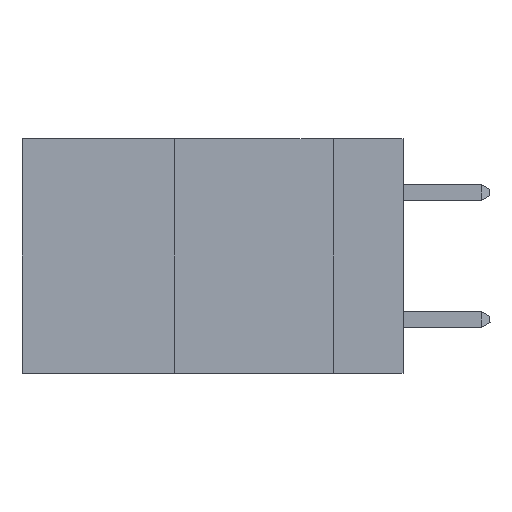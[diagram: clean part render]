
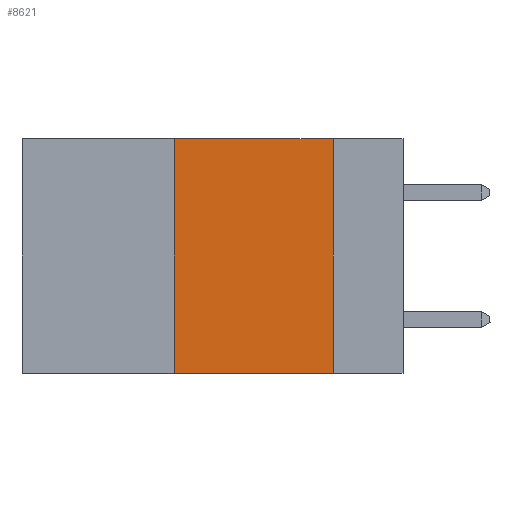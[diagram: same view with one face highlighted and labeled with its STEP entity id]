
A CAD part, left-side view. The second image highlights one B-rep face of the part: STEP entity #8621.
In plain terms, the highlighted planar face has unit normal (-1, 0, 0).
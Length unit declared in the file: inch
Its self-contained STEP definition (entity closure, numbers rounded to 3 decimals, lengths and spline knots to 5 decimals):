
#518 = PLANE ( 'NONE',  #20200 ) ;
#984 = DIRECTION ( 'NONE',  ( 0., 0., -1. ) ) ;
#2273 = VERTEX_POINT ( 'NONE', #17523 ) ;
#2694 = CARTESIAN_POINT ( 'NONE',  ( 0., 0.6, 0. ) ) ;
#3157 = ORIENTED_EDGE ( 'NONE', *, *, #17627, .T. ) ;
#3176 = EDGE_CURVE ( 'NONE', #18622, #2273, #8503, .T. ) ;
#4816 = DIRECTION ( 'NONE',  ( 0., 0., -1. ) ) ;
#5824 = EDGE_LOOP ( 'NONE', ( #12019, #20314, #16733, #3157 ) ) ;
#5862 = CARTESIAN_POINT ( 'NONE',  ( 0., 0.6, -0.37 ) ) ;
#7335 = LINE ( 'NONE', #13555, #12203 ) ;
#8503 = LINE ( 'NONE', #16429, #12730 ) ;
#8621 = ADVANCED_FACE ( 'NONE', ( #9488 ), #518, .F. ) ;
#9488 = FACE_OUTER_BOUND ( 'NONE', #5824, .T. ) ;
#10022 = VECTOR ( 'NONE', #26691, 39.37008 ) ;
#12019 = ORIENTED_EDGE ( 'NONE', *, *, #26061, .F. ) ;
#12203 = VECTOR ( 'NONE', #984, 39.37008 ) ;
#12730 = VECTOR ( 'NONE', #18592, 39.37008 ) ;
#13555 = CARTESIAN_POINT ( 'NONE',  ( 0., 0.11, 0. ) ) ;
#14818 = CARTESIAN_POINT ( 'NONE',  ( 0., 0.11, -0.37 ) ) ;
#15935 = VECTOR ( 'NONE', #19477, 39.37008 ) ;
#16429 = CARTESIAN_POINT ( 'NONE',  ( 0., 0.6, 0. ) ) ;
#16733 = ORIENTED_EDGE ( 'NONE', *, *, #23285, .F. ) ;
#17330 = DIRECTION ( 'NONE',  ( 1., 0., 0. ) ) ;
#17337 = CARTESIAN_POINT ( 'NONE',  ( 0., 0.36, 0. ) ) ;
#17523 = CARTESIAN_POINT ( 'NONE',  ( 0., 0.11, 0. ) ) ;
#17627 = EDGE_CURVE ( 'NONE', #23987, #26422, #26746, .T. ) ;
#18482 = CARTESIAN_POINT ( 'NONE',  ( 0., 0.36, 0. ) ) ;
#18592 = DIRECTION ( 'NONE',  ( 0., -1., 0. ) ) ;
#18622 = VERTEX_POINT ( 'NONE', #18482 ) ;
#19477 = DIRECTION ( 'NONE',  ( 0., 0., 1. ) ) ;
#19930 = CARTESIAN_POINT ( 'NONE',  ( 0., 0.36, -0.37 ) ) ;
#20200 = AXIS2_PLACEMENT_3D ( 'NONE', #2694, #17330, #4816 ) ;
#20314 = ORIENTED_EDGE ( 'NONE', *, *, #3176, .F. ) ;
#23285 = EDGE_CURVE ( 'NONE', #23987, #18622, #27087, .T. ) ;
#23987 = VERTEX_POINT ( 'NONE', #19930 ) ;
#26061 = EDGE_CURVE ( 'NONE', #2273, #26422, #7335, .T. ) ;
#26422 = VERTEX_POINT ( 'NONE', #14818 ) ;
#26691 = DIRECTION ( 'NONE',  ( 0., -1., 0. ) ) ;
#26746 = LINE ( 'NONE', #5862, #10022 ) ;
#27087 = LINE ( 'NONE', #17337, #15935 ) ;
